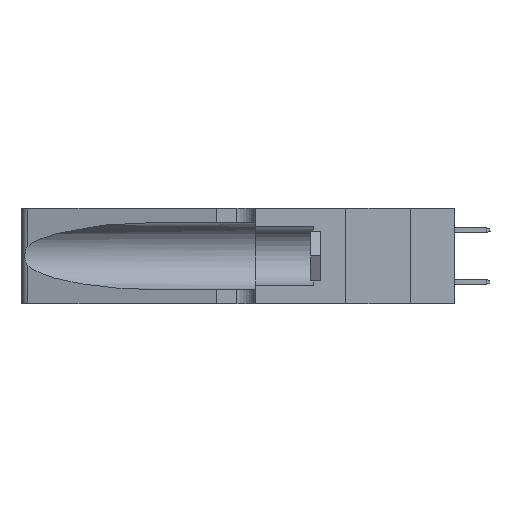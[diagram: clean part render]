
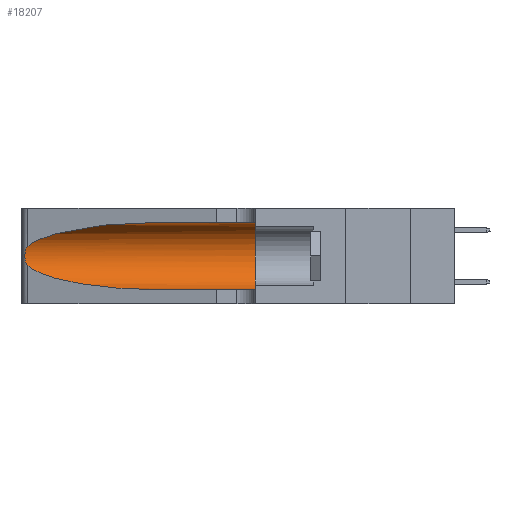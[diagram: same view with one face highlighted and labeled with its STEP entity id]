
A CAD part, left-side view. The second image highlights one B-rep face of the part: STEP entity #18207.
In plain terms, the highlighted cylindrical face has radius 3.308 mm (diameter 6.617 mm), a partial arc.
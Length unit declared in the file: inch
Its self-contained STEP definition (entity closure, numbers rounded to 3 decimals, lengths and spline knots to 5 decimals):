
#112 = CYLINDRICAL_SURFACE ( 'NONE', #33027, 0.13025 ) ;
#453 = CARTESIAN_POINT ( 'NONE',  ( 0.1305, 0.35, 0.31525 ) ) ;
#587 = CARTESIAN_POINT ( 'NONE',  ( 0.26075, 1.23896, 0.19203 ) ) ;
#883 = CARTESIAN_POINT ( 'NONE',  ( 0.18966, 0.96281, 0.31525 ) ) ;
#1861 = EDGE_CURVE ( 'NONE', #37463, #27878, #18115, .T. ) ;
#1964 = CARTESIAN_POINT ( 'NONE',  ( 0.1305, 0.72297, 0.31525 ) ) ;
#2619 = DIRECTION ( 'NONE',  ( 0., 1., 0. ) ) ;
#3169 = ORIENTED_EDGE ( 'NONE', *, *, #32767, .T. ) ;
#4112 = CARTESIAN_POINT ( 'NONE',  ( 0.25787, 1.23484, 0.2124 ) ) ;
#4188 = CARTESIAN_POINT ( 'NONE',  ( 0.25487, 1.22718, 0.14631 ) ) ;
#4607 = CARTESIAN_POINT ( 'NONE',  ( 0.1305, 0.72297, 0.31525 ) ) ;
#4855 = EDGE_CURVE ( 'NONE', #27878, #30157, #14114, .T. ) ;
#6846 = ORIENTED_EDGE ( 'NONE', *, *, #10379, .T. ) ;
#8195 = VERTEX_POINT ( 'NONE', #4188 ) ;
#8316 = DIRECTION ( 'NONE',  ( 0., -1., 0. ) ) ;
#9849 = CARTESIAN_POINT ( 'NONE',  ( 0.1305, 0.72297, 0.05475 ) ) ;
#9864 = CARTESIAN_POINT ( 'NONE',  ( 0.1305, 0.35, 0.05475 ) ) ;
#10379 = EDGE_CURVE ( 'NONE', #42674, #30157, #35399, .T. ) ;
#10522 = EDGE_CURVE ( 'NONE', #8195, #42674, #34246, .T. ) ;
#11216 = CARTESIAN_POINT ( 'NONE',  ( 0.26017, 1.23833, 0.17102 ) ) ;
#11446 = CARTESIAN_POINT ( 'NONE',  ( 0.25789, 1.23486, 0.15765 ) ) ;
#13167 = CARTESIAN_POINT ( 'NONE',  ( 0.18966, 0.96281, 0.05475 ) ) ;
#14071 = CARTESIAN_POINT ( 'NONE',  ( 0.26075, 1.23896, 0.178 ) ) ;
#14114 = CIRCLE ( 'NONE', #28966, 0.13025 ) ;
#14726 = CARTESIAN_POINT ( 'NONE',  ( 0.25555, 1.22993, 0.14849 ) ) ;
#16842 = B_SPLINE_CURVE_WITH_KNOTS ( 'NONE', 3,
 ( #43405, #34949, #34506, #4112, #17857, #37848, #587, #14071, #11216, #27633, #11446, #31407, #14726, #21623 ),
 .UNSPECIFIED., .F., .F.,
 ( 4, 2, 2, 2, 2, 2, 4 ),
 ( 0., 0.00027, 0.00053, 0.00107, 0.0016, 0.00187, 0.00214 ),
 .UNSPECIFIED. ) ;
#17857 = CARTESIAN_POINT ( 'NONE',  ( 0.25854, 1.2359, 0.20912 ) ) ;
#17896 = ORIENTED_EDGE ( 'NONE', *, *, #1861, .F. ) ;
#18115 = LINE ( 'NONE', #21235, #40587 ) ;
#18207 = ADVANCED_FACE ( 'NONE', ( #34029 ), #112, .F. ) ;
#18741 = CARTESIAN_POINT ( 'NONE',  ( 0.1305, 1.61858, 0.05475 ) ) ;
#20478 = EDGE_LOOP ( 'NONE', ( #3169, #26080, #28040, #6846, #28985, #17896 ) ) ;
#21235 = CARTESIAN_POINT ( 'NONE',  ( 0.1305, 1.61858, 0.31525 ) ) ;
#21623 = CARTESIAN_POINT ( 'NONE',  ( 0.25487, 1.22718, 0.14631 ) ) ;
#23615 = DIRECTION ( 'NONE',  ( 0., -1., 0. ) ) ;
#26080 = ORIENTED_EDGE ( 'NONE', *, *, #26950, .T. ) ;
#26950 = EDGE_CURVE ( 'NONE', #28240, #8195, #16842, .T. ) ;
#27633 = CARTESIAN_POINT ( 'NONE',  ( 0.25856, 1.23593, 0.16098 ) ) ;
#27878 = VERTEX_POINT ( 'NONE', #453 ) ;
#28040 = ORIENTED_EDGE ( 'NONE', *, *, #10522, .T. ) ;
#28240 = VERTEX_POINT ( 'NONE', #29654 ) ;
#28966 = AXIS2_PLACEMENT_3D ( 'NONE', #36744, #2619, #32997 ) ;
#28985 = ORIENTED_EDGE ( 'NONE', *, *, #4855, .F. ) ;
#29654 = CARTESIAN_POINT ( 'NONE',  ( 0.25487, 1.22718, 0.22369 ) ) ;
#30157 = VERTEX_POINT ( 'NONE', #9864 ) ;
#30236 = CARTESIAN_POINT ( 'NONE',  ( 0.1305, 1.61858, 0.185 ) ) ;
#30466 = DIRECTION ( 'NONE',  ( 0., 0., -1. ) ) ;
#31407 = CARTESIAN_POINT ( 'NONE',  ( 0.25639, 1.23186, 0.15144 ) ) ;
#32767 = EDGE_CURVE ( 'NONE', #37463, #28240, #38802, .T. ) ;
#32951 = CARTESIAN_POINT ( 'NONE',  ( 0.2373, 1.15595, 0.08982 ) ) ;
#32997 = DIRECTION ( 'NONE',  ( 0., 0., 1. ) ) ;
#33027 = AXIS2_PLACEMENT_3D ( 'NONE', #30236, #23615, #30466 ) ;
#34029 = FACE_OUTER_BOUND ( 'NONE', #20478, .T. ) ;
#34246 =( BOUNDED_CURVE ( )  B_SPLINE_CURVE ( 3, ( #43371, #32951, #13167, #9849 ),
 .UNSPECIFIED., .F., .T. ) 
 B_SPLINE_CURVE_WITH_KNOTS ( ( 4, 4 ),
 ( 3.44316, 4.71239 ),
 .UNSPECIFIED. ) 
 CURVE ( )  GEOMETRIC_REPRESENTATION_ITEM ( )  RATIONAL_B_SPLINE_CURVE ( ( 1., 0.87, 0.87, 1. ) ) 
 REPRESENTATION_ITEM ( '' )  );
#34506 = CARTESIAN_POINT ( 'NONE',  ( 0.25639, 1.23184, 0.21858 ) ) ;
#34569 = CARTESIAN_POINT ( 'NONE',  ( 0.25487, 1.22718, 0.22369 ) ) ;
#34949 = CARTESIAN_POINT ( 'NONE',  ( 0.25555, 1.22994, 0.2215 ) ) ;
#35399 = LINE ( 'NONE', #18741, #37766 ) ;
#36744 = CARTESIAN_POINT ( 'NONE',  ( 0.1305, 0.35, 0.185 ) ) ;
#37463 = VERTEX_POINT ( 'NONE', #1964 ) ;
#37766 = VECTOR ( 'NONE', #8316, 39.37008 ) ;
#37848 = CARTESIAN_POINT ( 'NONE',  ( 0.26018, 1.23835, 0.19895 ) ) ;
#38127 = CARTESIAN_POINT ( 'NONE',  ( 0.2373, 1.15595, 0.28018 ) ) ;
#38802 =( BOUNDED_CURVE ( )  B_SPLINE_CURVE ( 3, ( #4607, #883, #38127, #34569 ),
 .UNSPECIFIED., .F., .T. ) 
 B_SPLINE_CURVE_WITH_KNOTS ( ( 4, 4 ),
 ( 1.5708, 2.84003 ),
 .UNSPECIFIED. ) 
 CURVE ( )  GEOMETRIC_REPRESENTATION_ITEM ( )  RATIONAL_B_SPLINE_CURVE ( ( 1., 0.87, 0.87, 1. ) ) 
 REPRESENTATION_ITEM ( '' )  );
#40587 = VECTOR ( 'NONE', #42309, 39.37008 ) ;
#42309 = DIRECTION ( 'NONE',  ( 0., -1., 0. ) ) ;
#42674 = VERTEX_POINT ( 'NONE', #42865 ) ;
#42865 = CARTESIAN_POINT ( 'NONE',  ( 0.1305, 0.72297, 0.05475 ) ) ;
#43371 = CARTESIAN_POINT ( 'NONE',  ( 0.25487, 1.22718, 0.14631 ) ) ;
#43405 = CARTESIAN_POINT ( 'NONE',  ( 0.25487, 1.22718, 0.22369 ) ) ;
